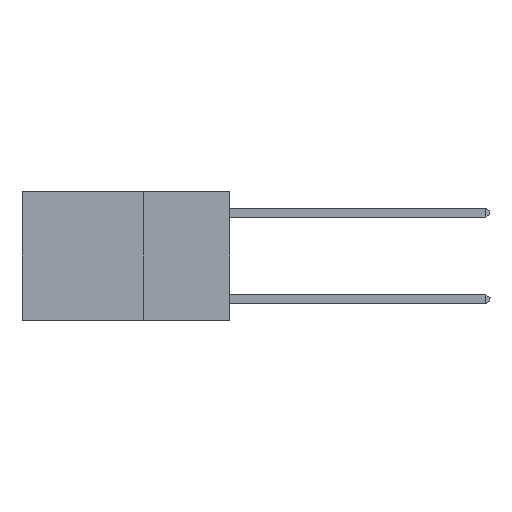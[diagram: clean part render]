
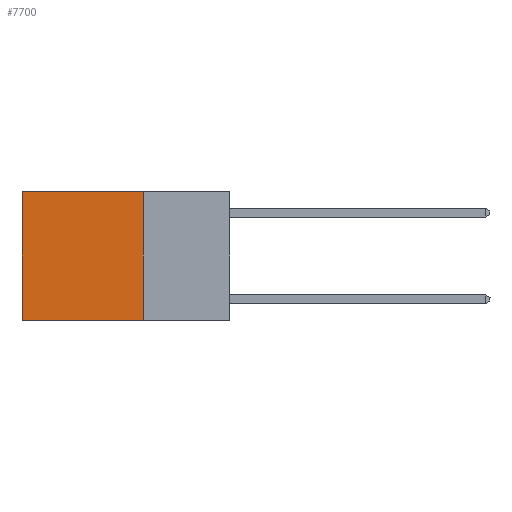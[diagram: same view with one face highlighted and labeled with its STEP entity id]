
A CAD part, left-side view. The second image highlights one B-rep face of the part: STEP entity #7700.
In plain terms, the highlighted planar face has unit normal (-1, 0, 0).
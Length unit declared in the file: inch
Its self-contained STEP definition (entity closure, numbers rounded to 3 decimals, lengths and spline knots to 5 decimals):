
#132 = ORIENTED_EDGE ( 'NONE', *, *, #25312, .T. ) ;
#837 = VECTOR ( 'NONE', #18975, 39.37008 ) ;
#1207 = DIRECTION ( 'NONE',  ( 1., 0., 0. ) ) ;
#1528 = FACE_OUTER_BOUND ( 'NONE', #13517, .T. ) ;
#2785 = LINE ( 'NONE', #5920, #21996 ) ;
#3976 = CARTESIAN_POINT ( 'NONE',  ( 0.2625, 0.25, 0. ) ) ;
#4525 = VERTEX_POINT ( 'NONE', #12606 ) ;
#5920 = CARTESIAN_POINT ( 'NONE',  ( 0.2625, 0.6, 0. ) ) ;
#6152 = VERTEX_POINT ( 'NONE', #24448 ) ;
#6223 = LINE ( 'NONE', #7083, #837 ) ;
#6973 = LINE ( 'NONE', #3976, #20828 ) ;
#7083 = CARTESIAN_POINT ( 'NONE',  ( 0.2625, 0.25, -0.37 ) ) ;
#7582 = VERTEX_POINT ( 'NONE', #18732 ) ;
#7700 = ADVANCED_FACE ( 'NONE', ( #1528 ), #19206, .F. ) ;
#8542 = VECTOR ( 'NONE', #9841, 39.37008 ) ;
#8760 = EDGE_CURVE ( 'NONE', #4525, #7582, #6223, .T. ) ;
#9841 = DIRECTION ( 'NONE',  ( 0., 1., 0. ) ) ;
#10647 = VERTEX_POINT ( 'NONE', #22927 ) ;
#10746 = ORIENTED_EDGE ( 'NONE', *, *, #24610, .F. ) ;
#11362 = AXIS2_PLACEMENT_3D ( 'NONE', #17328, #1207, #21084 ) ;
#12135 = DIRECTION ( 'NONE',  ( 0., 0., -1. ) ) ;
#12606 = CARTESIAN_POINT ( 'NONE',  ( 0.2625, 0.25, -0.37 ) ) ;
#13517 = EDGE_LOOP ( 'NONE', ( #13644, #17722, #10746, #132 ) ) ;
#13644 = ORIENTED_EDGE ( 'NONE', *, *, #24540, .T. ) ;
#17328 = CARTESIAN_POINT ( 'NONE',  ( 0.2625, 0.25, 0. ) ) ;
#17722 = ORIENTED_EDGE ( 'NONE', *, *, #8760, .F. ) ;
#18732 = CARTESIAN_POINT ( 'NONE',  ( 0.2625, 0.6, -0.37 ) ) ;
#18975 = DIRECTION ( 'NONE',  ( 0., 1., 0. ) ) ;
#19206 = PLANE ( 'NONE',  #11362 ) ;
#19945 = DIRECTION ( 'NONE',  ( 0., 0., -1. ) ) ;
#20828 = VECTOR ( 'NONE', #19945, 39.37008 ) ;
#21084 = DIRECTION ( 'NONE',  ( 0., 0., -1. ) ) ;
#21484 = CARTESIAN_POINT ( 'NONE',  ( 0.2625, 0.25, 0. ) ) ;
#21996 = VECTOR ( 'NONE', #12135, 39.37008 ) ;
#22827 = LINE ( 'NONE', #21484, #8542 ) ;
#22927 = CARTESIAN_POINT ( 'NONE',  ( 0.2625, 0.6, 0. ) ) ;
#24448 = CARTESIAN_POINT ( 'NONE',  ( 0.2625, 0.25, 0. ) ) ;
#24540 = EDGE_CURVE ( 'NONE', #10647, #7582, #2785, .T. ) ;
#24610 = EDGE_CURVE ( 'NONE', #6152, #4525, #6973, .T. ) ;
#25312 = EDGE_CURVE ( 'NONE', #6152, #10647, #22827, .T. ) ;
